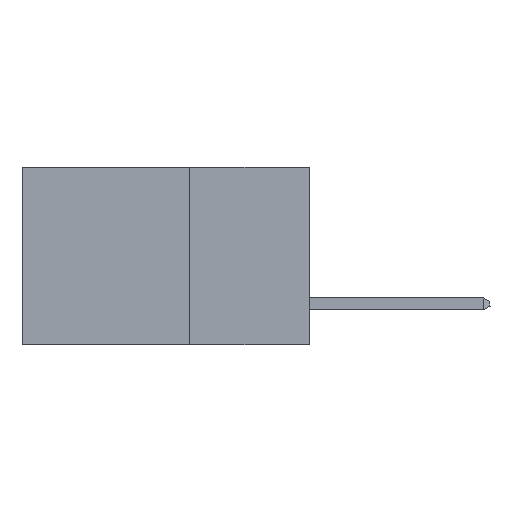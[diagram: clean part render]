
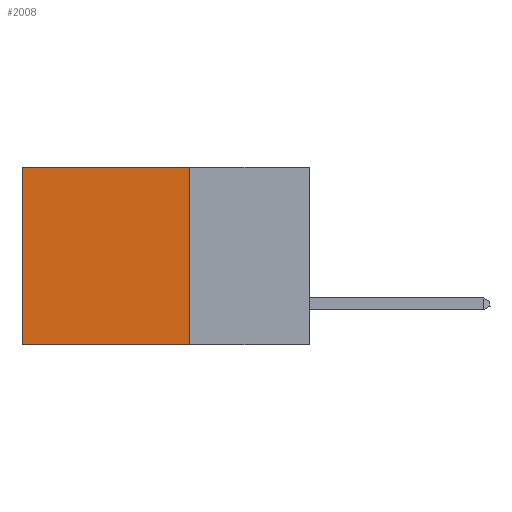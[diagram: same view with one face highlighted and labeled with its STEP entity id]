
A CAD part, left-side view. The second image highlights one B-rep face of the part: STEP entity #2008.
In plain terms, the highlighted planar face has unit normal (-1, 0, 0).
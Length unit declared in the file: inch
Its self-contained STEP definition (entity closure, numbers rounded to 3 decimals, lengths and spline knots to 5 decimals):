
#528 = AXIS2_PLACEMENT_3D ( 'NONE', #6223, #6323, #18652 ) ;
#844 = VERTEX_POINT ( 'NONE', #12275 ) ;
#1621 = LINE ( 'NONE', #12500, #8434 ) ;
#2008 = ADVANCED_FACE ( 'NONE', ( #13939 ), #17426, .F. ) ;
#2249 = CARTESIAN_POINT ( 'NONE',  ( 0.2875, 0.25, 0. ) ) ;
#4197 = LINE ( 'NONE', #2249, #4773 ) ;
#4696 = LINE ( 'NONE', #15297, #14275 ) ;
#4773 = VECTOR ( 'NONE', #10460, 39.37008 ) ;
#5667 = DIRECTION ( 'NONE',  ( 0., 1., 0. ) ) ;
#6223 = CARTESIAN_POINT ( 'NONE',  ( 0.2875, 0.25, 0. ) ) ;
#6323 = DIRECTION ( 'NONE',  ( 1., 0., 0. ) ) ;
#6959 = ORIENTED_EDGE ( 'NONE', *, *, #11103, .T. ) ;
#8434 = VECTOR ( 'NONE', #10964, 39.37008 ) ;
#8968 = CARTESIAN_POINT ( 'NONE',  ( 0.2875, 0.25, -0.37 ) ) ;
#9019 = VERTEX_POINT ( 'NONE', #18519 ) ;
#9225 = DIRECTION ( 'NONE',  ( 0., 0., -1. ) ) ;
#9434 = ORIENTED_EDGE ( 'NONE', *, *, #19301, .F. ) ;
#9756 = EDGE_CURVE ( 'NONE', #13849, #844, #4197, .T. ) ;
#10460 = DIRECTION ( 'NONE',  ( 0., 1., 0. ) ) ;
#10964 = DIRECTION ( 'NONE',  ( 0., 0., -1. ) ) ;
#11103 = EDGE_CURVE ( 'NONE', #844, #17713, #1621, .T. ) ;
#12127 = LINE ( 'NONE', #8968, #14830 ) ;
#12275 = CARTESIAN_POINT ( 'NONE',  ( 0.2875, 0.6, 0. ) ) ;
#12500 = CARTESIAN_POINT ( 'NONE',  ( 0.2875, 0.6, 0. ) ) ;
#13849 = VERTEX_POINT ( 'NONE', #19582 ) ;
#13939 = FACE_OUTER_BOUND ( 'NONE', #17721, .T. ) ;
#14275 = VECTOR ( 'NONE', #9225, 39.37008 ) ;
#14830 = VECTOR ( 'NONE', #5667, 39.37008 ) ;
#15159 = CARTESIAN_POINT ( 'NONE',  ( 0.2875, 0.6, -0.37 ) ) ;
#15297 = CARTESIAN_POINT ( 'NONE',  ( 0.2875, 0.25, 0. ) ) ;
#16769 = EDGE_CURVE ( 'NONE', #9019, #17713, #12127, .T. ) ;
#17296 = ORIENTED_EDGE ( 'NONE', *, *, #16769, .F. ) ;
#17426 = PLANE ( 'NONE',  #528 ) ;
#17713 = VERTEX_POINT ( 'NONE', #15159 ) ;
#17721 = EDGE_LOOP ( 'NONE', ( #6959, #17296, #9434, #17916 ) ) ;
#17916 = ORIENTED_EDGE ( 'NONE', *, *, #9756, .T. ) ;
#18519 = CARTESIAN_POINT ( 'NONE',  ( 0.2875, 0.25, -0.37 ) ) ;
#18652 = DIRECTION ( 'NONE',  ( 0., 0., -1. ) ) ;
#19301 = EDGE_CURVE ( 'NONE', #13849, #9019, #4696, .T. ) ;
#19582 = CARTESIAN_POINT ( 'NONE',  ( 0.2875, 0.25, 0. ) ) ;
